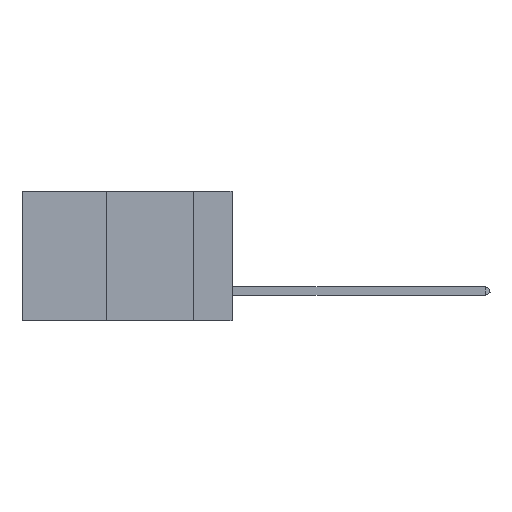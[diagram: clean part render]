
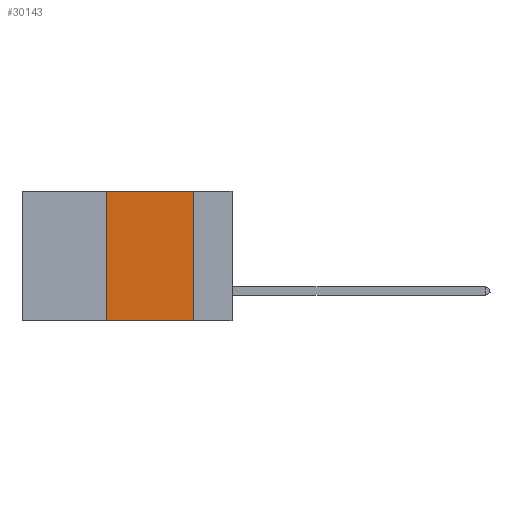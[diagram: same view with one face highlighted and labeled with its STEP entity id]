
A CAD part, left-side view. The second image highlights one B-rep face of the part: STEP entity #30143.
In plain terms, the highlighted planar face has unit normal (-1, 0, 0).
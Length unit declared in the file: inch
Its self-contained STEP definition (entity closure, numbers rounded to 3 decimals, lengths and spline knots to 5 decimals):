
#122 = LINE ( 'NONE', #9984, #26896 ) ;
#1013 = LINE ( 'NONE', #31493, #4949 ) ;
#1607 = CARTESIAN_POINT ( 'NONE',  ( 0., 0.11, -0.37 ) ) ;
#1799 = DIRECTION ( 'NONE',  ( 0., 0., -1. ) ) ;
#1960 = CARTESIAN_POINT ( 'NONE',  ( 0., 0.6, 0. ) ) ;
#3311 = CARTESIAN_POINT ( 'NONE',  ( 0., 0.6, 0. ) ) ;
#4607 = EDGE_CURVE ( 'NONE', #21604, #45387, #122, .T. ) ;
#4949 = VECTOR ( 'NONE', #45512, 39.37008 ) ;
#9984 = CARTESIAN_POINT ( 'NONE',  ( 0., 0.36, 0. ) ) ;
#12460 = CARTESIAN_POINT ( 'NONE',  ( 0., 0.11, 0. ) ) ;
#13094 = PLANE ( 'NONE',  #38838 ) ;
#14944 = DIRECTION ( 'NONE',  ( 0., 0., 1. ) ) ;
#15209 = VERTEX_POINT ( 'NONE', #1607 ) ;
#18270 = LINE ( 'NONE', #22049, #38192 ) ;
#19010 = DIRECTION ( 'NONE',  ( 0., -1., 0. ) ) ;
#20152 = VECTOR ( 'NONE', #28754, 39.37008 ) ;
#21604 = VERTEX_POINT ( 'NONE', #32684 ) ;
#21710 = ORIENTED_EDGE ( 'NONE', *, *, #40453, .T. ) ;
#22049 = CARTESIAN_POINT ( 'NONE',  ( 0., 0.6, -0.37 ) ) ;
#22573 = EDGE_LOOP ( 'NONE', ( #44061, #32977, #24285, #21710 ) ) ;
#22814 = EDGE_CURVE ( 'NONE', #45387, #28219, #42292, .T. ) ;
#23356 = FACE_OUTER_BOUND ( 'NONE', #22573, .T. ) ;
#23619 = DIRECTION ( 'NONE',  ( 1., 0., 0. ) ) ;
#24285 = ORIENTED_EDGE ( 'NONE', *, *, #4607, .F. ) ;
#26896 = VECTOR ( 'NONE', #14944, 39.37008 ) ;
#28219 = VERTEX_POINT ( 'NONE', #12460 ) ;
#28754 = DIRECTION ( 'NONE',  ( 0., -1., 0. ) ) ;
#30143 = ADVANCED_FACE ( 'NONE', ( #23356 ), #13094, .F. ) ;
#31493 = CARTESIAN_POINT ( 'NONE',  ( 0., 0.11, 0. ) ) ;
#32684 = CARTESIAN_POINT ( 'NONE',  ( 0., 0.36, -0.37 ) ) ;
#32977 = ORIENTED_EDGE ( 'NONE', *, *, #22814, .F. ) ;
#38192 = VECTOR ( 'NONE', #19010, 39.37008 ) ;
#38838 = AXIS2_PLACEMENT_3D ( 'NONE', #1960, #23619, #1799 ) ;
#40453 = EDGE_CURVE ( 'NONE', #21604, #15209, #18270, .T. ) ;
#42195 = EDGE_CURVE ( 'NONE', #28219, #15209, #1013, .T. ) ;
#42292 = LINE ( 'NONE', #3311, #20152 ) ;
#44061 = ORIENTED_EDGE ( 'NONE', *, *, #42195, .F. ) ;
#44660 = CARTESIAN_POINT ( 'NONE',  ( 0., 0.36, 0. ) ) ;
#45387 = VERTEX_POINT ( 'NONE', #44660 ) ;
#45512 = DIRECTION ( 'NONE',  ( 0., 0., -1. ) ) ;
